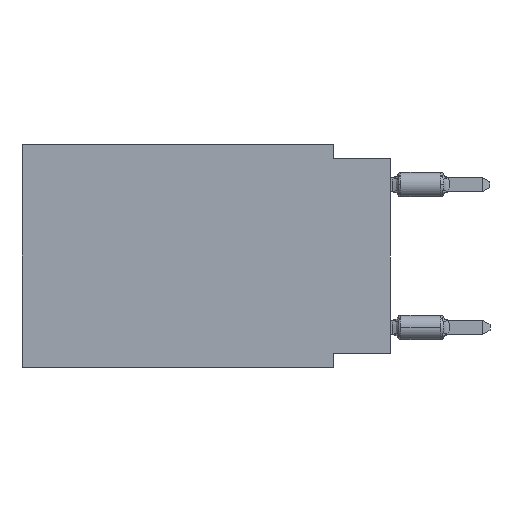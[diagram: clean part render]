
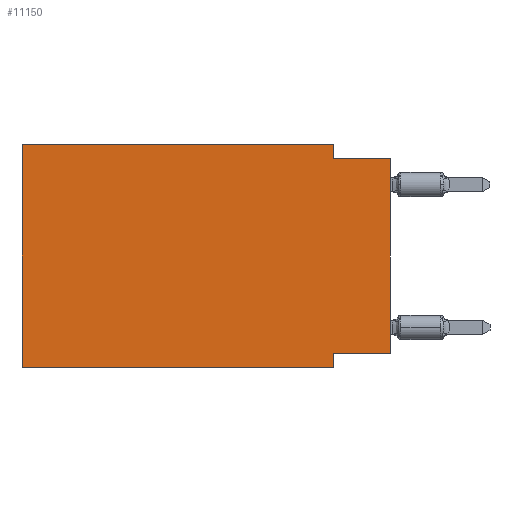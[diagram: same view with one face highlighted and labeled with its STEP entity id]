
A CAD part, left-side view. The second image highlights one B-rep face of the part: STEP entity #11150.
In plain terms, the highlighted planar face has unit normal (-1, 0, 0).
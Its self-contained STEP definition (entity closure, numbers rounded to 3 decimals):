
#279 = ORIENTED_EDGE ( 'NONE', *, *, #7240, .F. ) ;
#844 = LINE ( 'NONE', #13019, #13852 ) ;
#940 = EDGE_CURVE ( 'NONE', #13778, #9221, #17083, .T. ) ;
#980 = EDGE_CURVE ( 'NONE', #16941, #16608, #15964, .T. ) ;
#1240 = EDGE_LOOP ( 'NONE', ( #15319, #2835, #5591, #279, #16046, #6040, #15380, #7413 ) ) ;
#1311 = DIRECTION ( 'NONE',  ( 0., 1., 0. ) ) ;
#1457 = VECTOR ( 'NONE', #11980, 1000. ) ;
#1480 = EDGE_CURVE ( 'NONE', #14243, #16608, #13173, .T. ) ;
#2549 = LINE ( 'NONE', #8113, #11175 ) ;
#2672 = CARTESIAN_POINT ( 'NONE',  ( 0., 0., 0. ) ) ;
#2768 = DIRECTION ( 'NONE',  ( 0., 0., 1. ) ) ;
#2835 = ORIENTED_EDGE ( 'NONE', *, *, #1480, .F. ) ;
#3355 = VECTOR ( 'NONE', #1311, 1000. ) ;
#3404 = VECTOR ( 'NONE', #5273, 1000. ) ;
#4136 = VECTOR ( 'NONE', #9372, 1000. ) ;
#4902 = EDGE_CURVE ( 'NONE', #13778, #11334, #2549, .T. ) ;
#5269 = EDGE_CURVE ( 'NONE', #16941, #8695, #6701, .T. ) ;
#5273 = DIRECTION ( 'NONE',  ( 0., -1., 0. ) ) ;
#5468 = CARTESIAN_POINT ( 'NONE',  ( 0., 16.383, 0. ) ) ;
#5561 = DIRECTION ( 'NONE',  ( 0., 0., -1. ) ) ;
#5591 = ORIENTED_EDGE ( 'NONE', *, *, #6525, .F. ) ;
#6040 = ORIENTED_EDGE ( 'NONE', *, *, #4902, .T. ) ;
#6389 = CARTESIAN_POINT ( 'NONE',  ( 0., 0., -0.635 ) ) ;
#6525 = EDGE_CURVE ( 'NONE', #13980, #14243, #13908, .T. ) ;
#6701 = LINE ( 'NONE', #14778, #3355 ) ;
#6813 = DIRECTION ( 'NONE',  ( 0., -1., 0. ) ) ;
#7228 = EDGE_CURVE ( 'NONE', #8695, #11334, #844, .T. ) ;
#7240 = EDGE_CURVE ( 'NONE', #9221, #13980, #9276, .T. ) ;
#7413 = ORIENTED_EDGE ( 'NONE', *, *, #5269, .F. ) ;
#7796 = CARTESIAN_POINT ( 'NONE',  ( 0., 16.383, 0. ) ) ;
#8113 = CARTESIAN_POINT ( 'NONE',  ( 0., 16.383, -9.906 ) ) ;
#8536 = CARTESIAN_POINT ( 'NONE',  ( 0., 2.54, 0. ) ) ;
#8670 = VECTOR ( 'NONE', #2768, 1000. ) ;
#8695 = VERTEX_POINT ( 'NONE', #14896 ) ;
#9221 = VERTEX_POINT ( 'NONE', #11059 ) ;
#9276 = LINE ( 'NONE', #7796, #4136 ) ;
#9372 = DIRECTION ( 'NONE',  ( 0., -1., 0. ) ) ;
#9380 = FACE_OUTER_BOUND ( 'NONE', #1240, .T. ) ;
#10367 = CARTESIAN_POINT ( 'NONE',  ( 0., 2.54, -9.906 ) ) ;
#10603 = CARTESIAN_POINT ( 'NONE',  ( 0., 2.54, -0.635 ) ) ;
#11059 = CARTESIAN_POINT ( 'NONE',  ( 0., 16.383, 0. ) ) ;
#11140 = DIRECTION ( 'NONE',  ( 0., 0., -1. ) ) ;
#11150 = ADVANCED_FACE ( 'NONE', ( #9380 ), #14660, .F. ) ;
#11175 = VECTOR ( 'NONE', #6813, 1000. ) ;
#11302 = AXIS2_PLACEMENT_3D ( 'NONE', #12162, #11978, #5561 ) ;
#11334 = VERTEX_POINT ( 'NONE', #10367 ) ;
#11876 = CARTESIAN_POINT ( 'NONE',  ( 0., 0., -0.635 ) ) ;
#11978 = DIRECTION ( 'NONE',  ( 1., 0., 0. ) ) ;
#11980 = DIRECTION ( 'NONE',  ( 0., 0., 1. ) ) ;
#12162 = CARTESIAN_POINT ( 'NONE',  ( 0., 16.383, 0. ) ) ;
#12337 = VECTOR ( 'NONE', #11140, 1000. ) ;
#12536 = CARTESIAN_POINT ( 'NONE',  ( 0., 2.54, 0. ) ) ;
#13019 = CARTESIAN_POINT ( 'NONE',  ( 0., 2.54, -9.906 ) ) ;
#13173 = LINE ( 'NONE', #11876, #3404 ) ;
#13473 = CARTESIAN_POINT ( 'NONE',  ( 0., 0., -9.271 ) ) ;
#13778 = VERTEX_POINT ( 'NONE', #16001 ) ;
#13852 = VECTOR ( 'NONE', #17165, 1000. ) ;
#13908 = LINE ( 'NONE', #12536, #12337 ) ;
#13980 = VERTEX_POINT ( 'NONE', #8536 ) ;
#14243 = VERTEX_POINT ( 'NONE', #10603 ) ;
#14660 = PLANE ( 'NONE',  #11302 ) ;
#14778 = CARTESIAN_POINT ( 'NONE',  ( 0., 0., -9.271 ) ) ;
#14896 = CARTESIAN_POINT ( 'NONE',  ( 0., 2.54, -9.271 ) ) ;
#15319 = ORIENTED_EDGE ( 'NONE', *, *, #980, .T. ) ;
#15380 = ORIENTED_EDGE ( 'NONE', *, *, #7228, .F. ) ;
#15964 = LINE ( 'NONE', #2672, #8670 ) ;
#16001 = CARTESIAN_POINT ( 'NONE',  ( 0., 16.383, -9.906 ) ) ;
#16046 = ORIENTED_EDGE ( 'NONE', *, *, #940, .F. ) ;
#16608 = VERTEX_POINT ( 'NONE', #6389 ) ;
#16941 = VERTEX_POINT ( 'NONE', #13473 ) ;
#17083 = LINE ( 'NONE', #5468, #1457 ) ;
#17165 = DIRECTION ( 'NONE',  ( 0., 0., -1. ) ) ;
